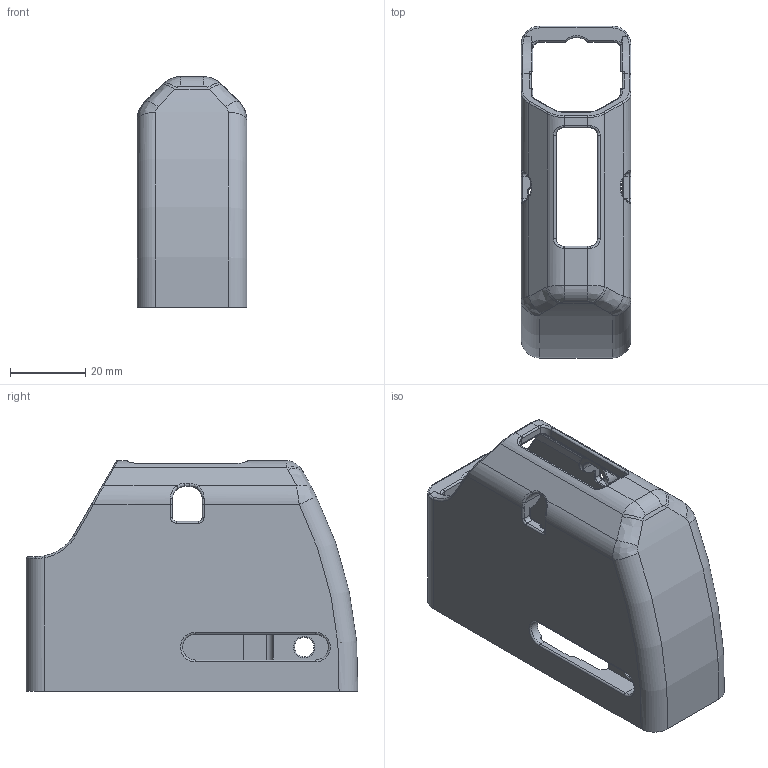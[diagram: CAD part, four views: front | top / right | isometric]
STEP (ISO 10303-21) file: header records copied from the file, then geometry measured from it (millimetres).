
FILE_DESCRIPTION(/* description */ (''),/* implementation_level */ '2;1');
FILE_NAME(/* name */ 'freeloader-body-milspec-magcatch-plain-v3.step',/* time_stamp */ '2021-09-20T14:44:46-07:00',/* author */ (''),/* organization */ (''),/* preprocessor_version */ 'ST-DEVELOPER v18.1',/* originating_system */ 'Autodesk Translation Framework v10.10.0.1391',/* authorisation */ '');
FILE_SCHEMA (('AUTOMOTIVE_DESIGN { 1 0 10303 214 3 1 1 }'));
Length unit declared in the file: millimetre
Products named in the file (1): loader-base-v0.3_magcatch_plain
Bounding box: 29.22 x 88.21 x 61.31 mm (x, y, z)
Volume: 46817 mm3; surface area: 23898.8 mm2
Topology: 1 solids, 1 shells, 374 faces, 953 edges, 574 vertices
Faces by surface type: cylinder 127, plane 100, bspline 82, torus 63, cone 2
Full cylindrical faces by diameter (mm): 5.182 x1, 7.925 x1
Entity records: 13870 total; most frequent: CARTESIAN_POINT 5070, ORIENTED_EDGE 1904, DIRECTION 1790, EDGE_CURVE 952, AXIS2_PLACEMENT_3D 707, VERTEX_POINT 574, EDGE_LOOP 380, LINE 376
